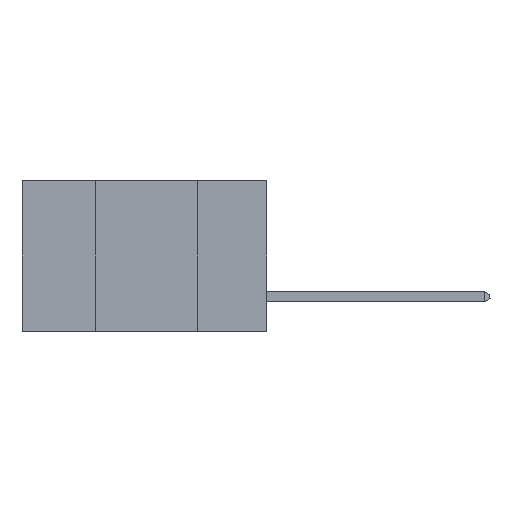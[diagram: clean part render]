
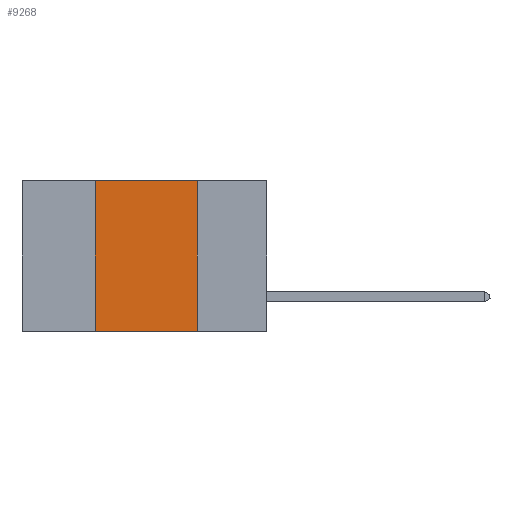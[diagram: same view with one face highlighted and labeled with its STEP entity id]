
A CAD part, left-side view. The second image highlights one B-rep face of the part: STEP entity #9268.
In plain terms, the highlighted planar face has unit normal (-1, 0, 0).
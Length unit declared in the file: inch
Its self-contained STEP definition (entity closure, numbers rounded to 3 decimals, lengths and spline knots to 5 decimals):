
#4628 = EDGE_CURVE ( 'NONE', #26876, #7344, #34414, .T. ) ;
#5627 = AXIS2_PLACEMENT_3D ( 'NONE', #22565, #15161, #7490 ) ;
#6396 = VERTEX_POINT ( 'NONE', #38582 ) ;
#6735 = DIRECTION ( 'NONE',  ( 0., -1., 0. ) ) ;
#6963 = EDGE_LOOP ( 'NONE', ( #35366, #33857, #13457, #46769 ) ) ;
#7344 = VERTEX_POINT ( 'NONE', #42421 ) ;
#7490 = DIRECTION ( 'NONE',  ( 0., 0., -1. ) ) ;
#7930 = VERTEX_POINT ( 'NONE', #18695 ) ;
#8628 = VECTOR ( 'NONE', #6735, 39.37008 ) ;
#9268 = ADVANCED_FACE ( 'NONE', ( #39906 ), #26714, .F. ) ;
#13457 = ORIENTED_EDGE ( 'NONE', *, *, #32966, .F. ) ;
#14543 = CARTESIAN_POINT ( 'NONE',  ( 0., 0.17, 0. ) ) ;
#14643 = CARTESIAN_POINT ( 'NONE',  ( 0., 0.42, -0.37 ) ) ;
#15161 = DIRECTION ( 'NONE',  ( 1., 0., 0. ) ) ;
#15393 = LINE ( 'NONE', #14543, #29784 ) ;
#18695 = CARTESIAN_POINT ( 'NONE',  ( 0., 0.17, 0. ) ) ;
#21194 = VECTOR ( 'NONE', #25429, 39.37008 ) ;
#22200 = VECTOR ( 'NONE', #22493, 39.37008 ) ;
#22493 = DIRECTION ( 'NONE',  ( 0., -1., 0. ) ) ;
#22565 = CARTESIAN_POINT ( 'NONE',  ( 0., 0.6, 0. ) ) ;
#23576 = EDGE_CURVE ( 'NONE', #6396, #7930, #27545, .T. ) ;
#24777 = CARTESIAN_POINT ( 'NONE',  ( 0., 0.42, 0. ) ) ;
#25292 = EDGE_CURVE ( 'NONE', #7930, #7344, #15393, .T. ) ;
#25429 = DIRECTION ( 'NONE',  ( 0., 0., 1. ) ) ;
#26714 = PLANE ( 'NONE',  #5627 ) ;
#26876 = VERTEX_POINT ( 'NONE', #14643 ) ;
#27545 = LINE ( 'NONE', #30678, #22200 ) ;
#29784 = VECTOR ( 'NONE', #30118, 39.37008 ) ;
#30118 = DIRECTION ( 'NONE',  ( 0., 0., -1. ) ) ;
#30678 = CARTESIAN_POINT ( 'NONE',  ( 0., 0.6, 0. ) ) ;
#30796 = LINE ( 'NONE', #24777, #21194 ) ;
#32966 = EDGE_CURVE ( 'NONE', #26876, #6396, #30796, .T. ) ;
#33857 = ORIENTED_EDGE ( 'NONE', *, *, #23576, .F. ) ;
#34414 = LINE ( 'NONE', #49207, #8628 ) ;
#35366 = ORIENTED_EDGE ( 'NONE', *, *, #25292, .F. ) ;
#38582 = CARTESIAN_POINT ( 'NONE',  ( 0., 0.42, 0. ) ) ;
#39906 = FACE_OUTER_BOUND ( 'NONE', #6963, .T. ) ;
#42421 = CARTESIAN_POINT ( 'NONE',  ( 0., 0.17, -0.37 ) ) ;
#46769 = ORIENTED_EDGE ( 'NONE', *, *, #4628, .T. ) ;
#49207 = CARTESIAN_POINT ( 'NONE',  ( 0., 0.6, -0.37 ) ) ;
